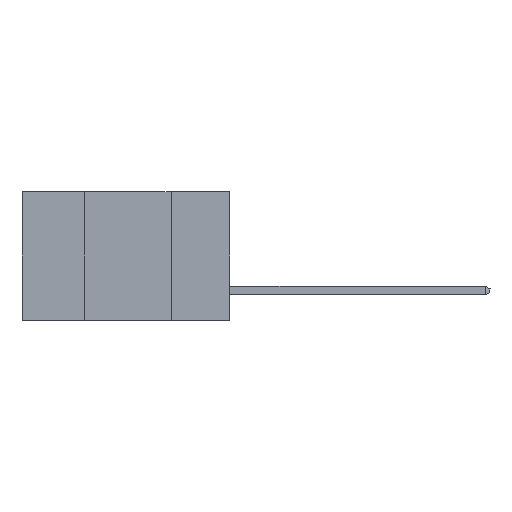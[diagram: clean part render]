
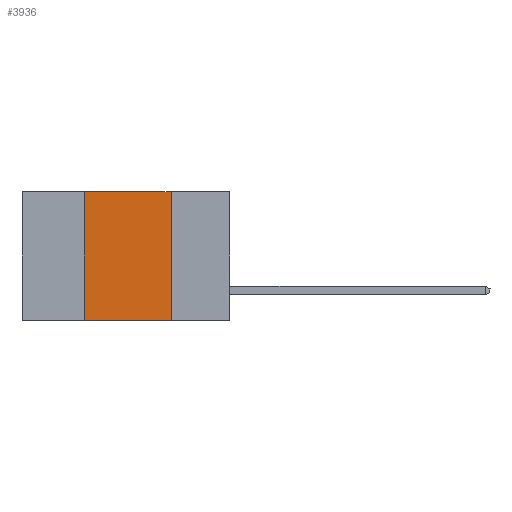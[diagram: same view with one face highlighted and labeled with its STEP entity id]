
A CAD part, left-side view. The second image highlights one B-rep face of the part: STEP entity #3936.
In plain terms, the highlighted planar face has unit normal (-1, 0, 0).
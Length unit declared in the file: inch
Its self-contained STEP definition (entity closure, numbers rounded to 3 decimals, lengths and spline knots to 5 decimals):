
#217 = CARTESIAN_POINT ( 'NONE',  ( 0., 0.42, -0.37 ) ) ;
#330 = EDGE_CURVE ( 'NONE', #3677, #7652, #782, .T. ) ;
#762 = VECTOR ( 'NONE', #5809, 39.37008 ) ;
#782 = LINE ( 'NONE', #4672, #12457 ) ;
#1276 = EDGE_CURVE ( 'NONE', #7652, #6050, #4271, .T. ) ;
#2030 = ORIENTED_EDGE ( 'NONE', *, *, #330, .F. ) ;
#2386 = LINE ( 'NONE', #4221, #3214 ) ;
#3214 = VECTOR ( 'NONE', #12164, 39.37008 ) ;
#3462 = EDGE_CURVE ( 'NONE', #7612, #6050, #3508, .T. ) ;
#3508 = LINE ( 'NONE', #5526, #6454 ) ;
#3677 = VERTEX_POINT ( 'NONE', #8820 ) ;
#3688 = DIRECTION ( 'NONE',  ( 1., 0., 0. ) ) ;
#3936 = ADVANCED_FACE ( 'NONE', ( #8683 ), #5577, .F. ) ;
#4221 = CARTESIAN_POINT ( 'NONE',  ( 0., 0.42, -0.37 ) ) ;
#4271 = LINE ( 'NONE', #11606, #762 ) ;
#4295 = DIRECTION ( 'NONE',  ( 0., -1., 0. ) ) ;
#4571 = CARTESIAN_POINT ( 'NONE',  ( 0., 0.17, 0. ) ) ;
#4672 = CARTESIAN_POINT ( 'NONE',  ( 0., 0.6, 0. ) ) ;
#4739 = DIRECTION ( 'NONE',  ( 0., -1., 0. ) ) ;
#5366 = ORIENTED_EDGE ( 'NONE', *, *, #8111, .F. ) ;
#5526 = CARTESIAN_POINT ( 'NONE',  ( 0., 0.6, -0.37 ) ) ;
#5577 = PLANE ( 'NONE',  #11190 ) ;
#5604 = ORIENTED_EDGE ( 'NONE', *, *, #1276, .F. ) ;
#5809 = DIRECTION ( 'NONE',  ( 0., 0., -1. ) ) ;
#6050 = VERTEX_POINT ( 'NONE', #10238 ) ;
#6454 = VECTOR ( 'NONE', #4295, 39.37008 ) ;
#7509 = DIRECTION ( 'NONE',  ( 0., 0., -1. ) ) ;
#7612 = VERTEX_POINT ( 'NONE', #217 ) ;
#7652 = VERTEX_POINT ( 'NONE', #4571 ) ;
#7702 = CARTESIAN_POINT ( 'NONE',  ( 0., 0.6, 0. ) ) ;
#8111 = EDGE_CURVE ( 'NONE', #7612, #3677, #2386, .T. ) ;
#8501 = ORIENTED_EDGE ( 'NONE', *, *, #3462, .T. ) ;
#8683 = FACE_OUTER_BOUND ( 'NONE', #11988, .T. ) ;
#8820 = CARTESIAN_POINT ( 'NONE',  ( 0., 0.42, 0. ) ) ;
#10238 = CARTESIAN_POINT ( 'NONE',  ( 0., 0.17, -0.37 ) ) ;
#11190 = AXIS2_PLACEMENT_3D ( 'NONE', #7702, #3688, #7509 ) ;
#11606 = CARTESIAN_POINT ( 'NONE',  ( 0., 0.17, -0.37 ) ) ;
#11988 = EDGE_LOOP ( 'NONE', ( #5604, #2030, #5366, #8501 ) ) ;
#12164 = DIRECTION ( 'NONE',  ( 0., 0., 1. ) ) ;
#12457 = VECTOR ( 'NONE', #4739, 39.37008 ) ;
